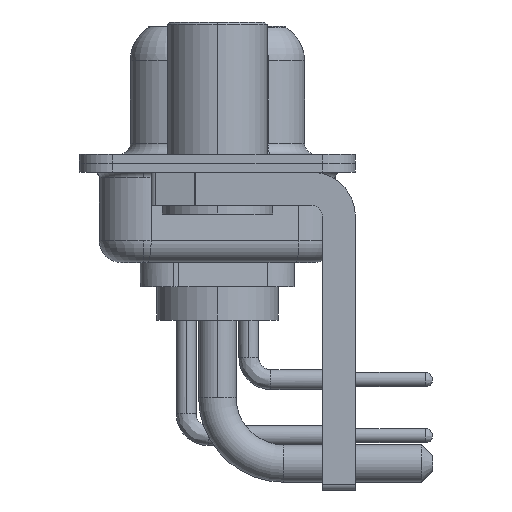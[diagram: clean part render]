
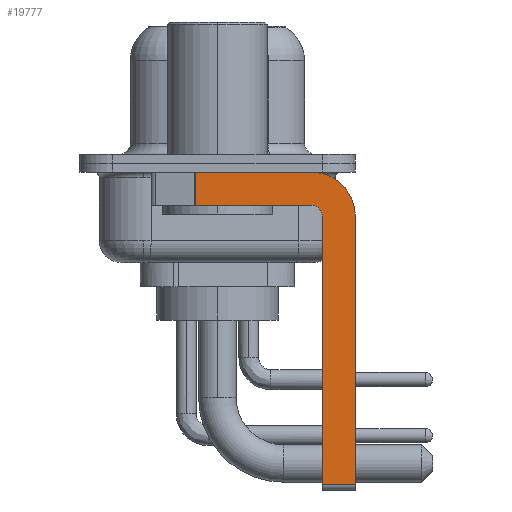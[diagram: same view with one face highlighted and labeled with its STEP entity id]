
A CAD part, left-side view. The second image highlights one B-rep face of the part: STEP entity #19777.
In plain terms, the highlighted planar face has unit normal (-1, 0, 0).
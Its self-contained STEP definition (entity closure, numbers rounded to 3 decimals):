
#31 = ORIENTED_EDGE ( 'NONE', *, *, #14557, .F. ) ;
#185 = LINE ( 'NONE', #470, #16830 ) ;
#271 = FACE_OUTER_BOUND ( 'NONE', #7058, .T. ) ;
#372 = VERTEX_POINT ( 'NONE', #18011 ) ;
#470 = CARTESIAN_POINT ( 'NONE',  ( -2.9, -4.75, -14.8 ) ) ;
#3381 = DIRECTION ( 'NONE',  ( 0., 1., 0. ) ) ;
#3501 = LINE ( 'NONE', #13207, #7423 ) ;
#4277 = EDGE_CURVE ( 'NONE', #18411, #5544, #7795, .T. ) ;
#4398 = CARTESIAN_POINT ( 'NONE',  ( -2.9, -4.25, -2.4 ) ) ;
#5001 = CARTESIAN_POINT ( 'NONE',  ( -2.9, 0.978, -0.4 ) ) ;
#5226 = AXIS2_PLACEMENT_3D ( 'NONE', #4398, #15089, #7489 ) ;
#5291 = ORIENTED_EDGE ( 'NONE', *, *, #11985, .F. ) ;
#5304 = DIRECTION ( 'NONE',  ( 0., 0., -1. ) ) ;
#5359 = CARTESIAN_POINT ( 'NONE',  ( -2.9, -4.75, -2.4 ) ) ;
#5410 = ORIENTED_EDGE ( 'NONE', *, *, #16847, .F. ) ;
#5544 = VERTEX_POINT ( 'NONE', #19549 ) ;
#5588 = ORIENTED_EDGE ( 'NONE', *, *, #14161, .F. ) ;
#5648 = CIRCLE ( 'NONE', #7876, 0.5 ) ;
#6879 = ORIENTED_EDGE ( 'NONE', *, *, #4277, .T. ) ;
#7058 = EDGE_LOOP ( 'NONE', ( #5291, #15604, #5588, #10279, #19750, #6879, #5410, #31 ) ) ;
#7364 = EDGE_CURVE ( 'NONE', #16346, #9220, #3501, .T. ) ;
#7384 = CARTESIAN_POINT ( 'NONE',  ( -2.9, -4.25, -2.4 ) ) ;
#7423 = VECTOR ( 'NONE', #8290, 1000. ) ;
#7489 = DIRECTION ( 'NONE',  ( 0., 0., -1. ) ) ;
#7795 = LINE ( 'NONE', #18421, #13440 ) ;
#7832 = VECTOR ( 'NONE', #12920, 1000. ) ;
#7876 = AXIS2_PLACEMENT_3D ( 'NONE', #7384, #13490, #13194 ) ;
#8290 = DIRECTION ( 'NONE',  ( 0., 0., -1. ) ) ;
#8545 = AXIS2_PLACEMENT_3D ( 'NONE', #19770, #18370, #12368 ) ;
#9220 = VERTEX_POINT ( 'NONE', #12780 ) ;
#9392 = DIRECTION ( 'NONE',  ( 0., -1., 0. ) ) ;
#9752 = VERTEX_POINT ( 'NONE', #5359 ) ;
#10279 = ORIENTED_EDGE ( 'NONE', *, *, #12725, .F. ) ;
#10696 = LINE ( 'NONE', #15581, #14301 ) ;
#11413 = LINE ( 'NONE', #19009, #14426 ) ;
#11633 = CARTESIAN_POINT ( 'NONE',  ( -2.9, 3., -0.4 ) ) ;
#11985 = EDGE_CURVE ( 'NONE', #16346, #14586, #13115, .T. ) ;
#12208 = CARTESIAN_POINT ( 'NONE',  ( -2.9, -4.75, -14.55 ) ) ;
#12368 = DIRECTION ( 'NONE',  ( 0., 0., -1. ) ) ;
#12675 = DIRECTION ( 'NONE',  ( 0., 0., 1. ) ) ;
#12725 = EDGE_CURVE ( 'NONE', #9752, #372, #5648, .T. ) ;
#12780 = CARTESIAN_POINT ( 'NONE',  ( -2.9, 0.978, -1.9 ) ) ;
#12883 = EDGE_CURVE ( 'NONE', #18411, #9752, #185, .T. ) ;
#12920 = DIRECTION ( 'NONE',  ( 0., -1., 0. ) ) ;
#13115 = LINE ( 'NONE', #11633, #7832 ) ;
#13194 = DIRECTION ( 'NONE',  ( 0., 0., 1. ) ) ;
#13207 = CARTESIAN_POINT ( 'NONE',  ( -2.9, 0.978, -1.9 ) ) ;
#13440 = VECTOR ( 'NONE', #9392, 1000. ) ;
#13490 = DIRECTION ( 'NONE',  ( -1., 0., 0. ) ) ;
#13759 = CARTESIAN_POINT ( 'NONE',  ( -2.9, -6.25, -2.4 ) ) ;
#14161 = EDGE_CURVE ( 'NONE', #372, #9220, #10696, .T. ) ;
#14301 = VECTOR ( 'NONE', #3381, 1000. ) ;
#14426 = VECTOR ( 'NONE', #5304, 1000. ) ;
#14557 = EDGE_CURVE ( 'NONE', #14586, #17479, #14607, .T. ) ;
#14586 = VERTEX_POINT ( 'NONE', #15350 ) ;
#14607 = CIRCLE ( 'NONE', #8545, 2. ) ;
#15089 = DIRECTION ( 'NONE',  ( 1., 0., 0. ) ) ;
#15350 = CARTESIAN_POINT ( 'NONE',  ( -2.9, -4.25, -0.4 ) ) ;
#15581 = CARTESIAN_POINT ( 'NONE',  ( -2.9, -4.25, -1.9 ) ) ;
#15604 = ORIENTED_EDGE ( 'NONE', *, *, #7364, .T. ) ;
#16346 = VERTEX_POINT ( 'NONE', #5001 ) ;
#16830 = VECTOR ( 'NONE', #12675, 1000. ) ;
#16847 = EDGE_CURVE ( 'NONE', #17479, #5544, #11413, .T. ) ;
#17479 = VERTEX_POINT ( 'NONE', #13759 ) ;
#18011 = CARTESIAN_POINT ( 'NONE',  ( -2.9, -4.25, -1.9 ) ) ;
#18101 = PLANE ( 'NONE',  #5226 ) ;
#18370 = DIRECTION ( 'NONE',  ( 1., 0., 0. ) ) ;
#18411 = VERTEX_POINT ( 'NONE', #12208 ) ;
#18421 = CARTESIAN_POINT ( 'NONE',  ( -2.9, -4.25, -14.55 ) ) ;
#19009 = CARTESIAN_POINT ( 'NONE',  ( -2.9, -6.25, -2.4 ) ) ;
#19549 = CARTESIAN_POINT ( 'NONE',  ( -2.9, -6.25, -14.55 ) ) ;
#19750 = ORIENTED_EDGE ( 'NONE', *, *, #12883, .F. ) ;
#19770 = CARTESIAN_POINT ( 'NONE',  ( -2.9, -4.25, -2.4 ) ) ;
#19777 = ADVANCED_FACE ( 'NONE', ( #271 ), #18101, .F. ) ;
